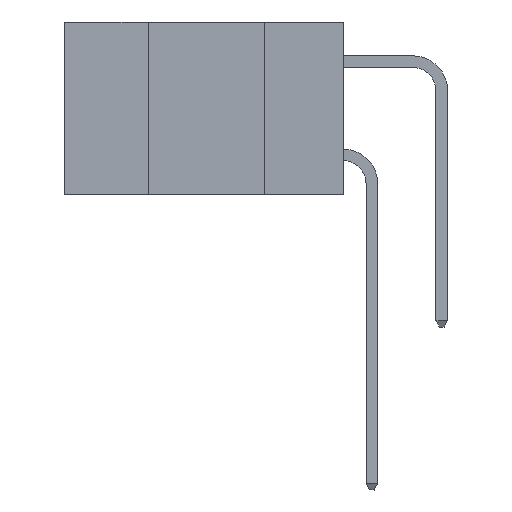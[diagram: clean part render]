
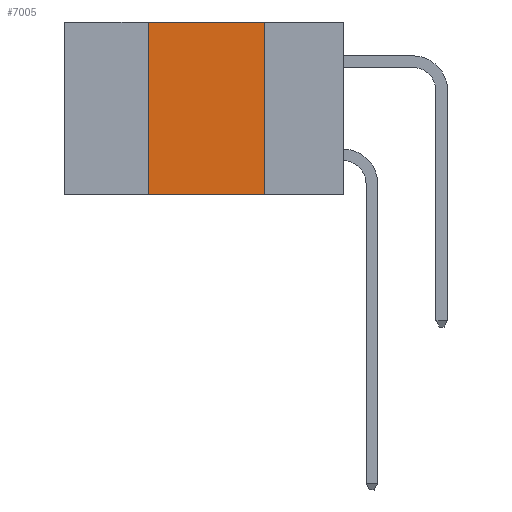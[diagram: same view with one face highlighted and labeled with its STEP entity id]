
A CAD part, left-side view. The second image highlights one B-rep face of the part: STEP entity #7005.
In plain terms, the highlighted planar face has unit normal (-1, 0, 0).
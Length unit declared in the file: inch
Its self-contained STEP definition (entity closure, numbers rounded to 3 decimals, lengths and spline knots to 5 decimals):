
#116 = CARTESIAN_POINT ( 'NONE',  ( 0., 0.17, 0. ) ) ;
#175 = VECTOR ( 'NONE', #12116, 39.37008 ) ;
#893 = DIRECTION ( 'NONE',  ( 0., -1., 0. ) ) ;
#1542 = DIRECTION ( 'NONE',  ( 0., 0., -1. ) ) ;
#1764 = CARTESIAN_POINT ( 'NONE',  ( 0., 0.17, -0.37 ) ) ;
#2037 = CARTESIAN_POINT ( 'NONE',  ( 0., 0.42, -0.37 ) ) ;
#2190 = CARTESIAN_POINT ( 'NONE',  ( 0., 0.6, 0. ) ) ;
#2560 = LINE ( 'NONE', #17838, #4915 ) ;
#2703 = ORIENTED_EDGE ( 'NONE', *, *, #3978, .F. ) ;
#3225 = AXIS2_PLACEMENT_3D ( 'NONE', #8537, #6890, #1542 ) ;
#3779 = LINE ( 'NONE', #2190, #175 ) ;
#3978 = EDGE_CURVE ( 'NONE', #14727, #4022, #3779, .T. ) ;
#4022 = VERTEX_POINT ( 'NONE', #116 ) ;
#4915 = VECTOR ( 'NONE', #893, 39.37008 ) ;
#5386 = VECTOR ( 'NONE', #12960, 39.37008 ) ;
#6158 = FACE_OUTER_BOUND ( 'NONE', #13847, .T. ) ;
#6890 = DIRECTION ( 'NONE',  ( 1., 0., 0. ) ) ;
#7005 = ADVANCED_FACE ( 'NONE', ( #6158 ), #14173, .F. ) ;
#7072 = ORIENTED_EDGE ( 'NONE', *, *, #8060, .F. ) ;
#7233 = CARTESIAN_POINT ( 'NONE',  ( 0., 0.17, -0.37 ) ) ;
#8060 = EDGE_CURVE ( 'NONE', #4022, #10925, #10395, .T. ) ;
#8537 = CARTESIAN_POINT ( 'NONE',  ( 0., 0.6, 0. ) ) ;
#10224 = CARTESIAN_POINT ( 'NONE',  ( 0., 0.42, -0.37 ) ) ;
#10395 = LINE ( 'NONE', #1764, #5386 ) ;
#10673 = LINE ( 'NONE', #2037, #11670 ) ;
#10842 = CARTESIAN_POINT ( 'NONE',  ( 0., 0.42, 0. ) ) ;
#10925 = VERTEX_POINT ( 'NONE', #7233 ) ;
#11670 = VECTOR ( 'NONE', #16244, 39.37008 ) ;
#12116 = DIRECTION ( 'NONE',  ( 0., -1., 0. ) ) ;
#12960 = DIRECTION ( 'NONE',  ( 0., 0., -1. ) ) ;
#13847 = EDGE_LOOP ( 'NONE', ( #7072, #2703, #15849, #13964 ) ) ;
#13964 = ORIENTED_EDGE ( 'NONE', *, *, #15197, .T. ) ;
#14091 = EDGE_CURVE ( 'NONE', #17388, #14727, #10673, .T. ) ;
#14173 = PLANE ( 'NONE',  #3225 ) ;
#14727 = VERTEX_POINT ( 'NONE', #10842 ) ;
#15197 = EDGE_CURVE ( 'NONE', #17388, #10925, #2560, .T. ) ;
#15849 = ORIENTED_EDGE ( 'NONE', *, *, #14091, .F. ) ;
#16244 = DIRECTION ( 'NONE',  ( 0., 0., 1. ) ) ;
#17388 = VERTEX_POINT ( 'NONE', #10224 ) ;
#17838 = CARTESIAN_POINT ( 'NONE',  ( 0., 0.6, -0.37 ) ) ;
